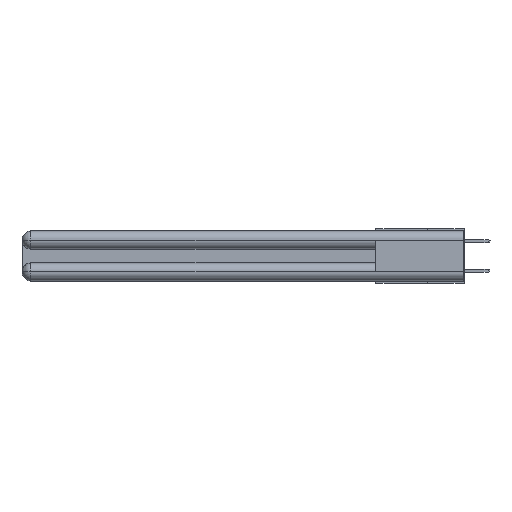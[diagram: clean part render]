
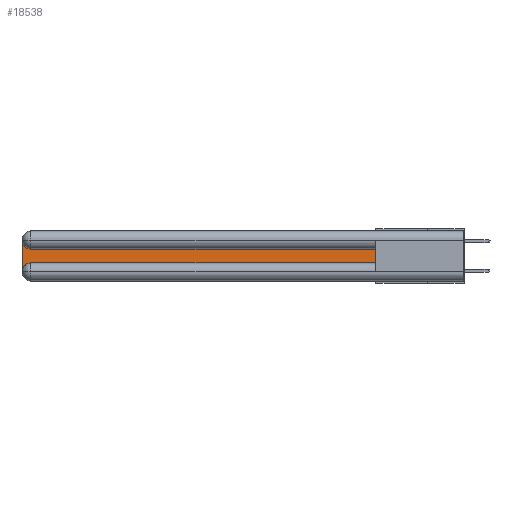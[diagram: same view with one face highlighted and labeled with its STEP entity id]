
A CAD part, left-side view. The second image highlights one B-rep face of the part: STEP entity #18538.
In plain terms, the highlighted planar face has unit normal (-1, 0, 0).
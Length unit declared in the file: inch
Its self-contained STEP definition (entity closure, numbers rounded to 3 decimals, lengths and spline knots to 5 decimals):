
#645 = EDGE_CURVE ( 'NONE', #24647, #4010, #3959, .T. ) ;
#1562 = VERTEX_POINT ( 'NONE', #2210 ) ;
#2210 = CARTESIAN_POINT ( 'NONE',  ( 0.075, 2.94, -0.1225 ) ) ;
#3118 = DIRECTION ( 'NONE',  ( 0., 1., 0. ) ) ;
#3959 = CIRCLE ( 'NONE', #5867, 0.06 ) ;
#4010 = VERTEX_POINT ( 'NONE', #17781 ) ;
#4594 = EDGE_CURVE ( 'NONE', #27675, #24647, #27883, .T. ) ;
#4763 = EDGE_CURVE ( 'NONE', #5570, #25290, #13779, .T. ) ;
#5570 = VERTEX_POINT ( 'NONE', #21222 ) ;
#5867 = AXIS2_PLACEMENT_3D ( 'NONE', #15861, #25127, #15965 ) ;
#6139 = CARTESIAN_POINT ( 'NONE',  ( 0.075, 0.6, -0.2175 ) ) ;
#8546 = VECTOR ( 'NONE', #24603, 39.37008 ) ;
#8799 = CARTESIAN_POINT ( 'NONE',  ( 0.075, 0.6, -0.2175 ) ) ;
#8911 = DIRECTION ( 'NONE',  ( 0., 0., -1. ) ) ;
#9016 = CARTESIAN_POINT ( 'NONE',  ( 0.075, 2.94, -0.0625 ) ) ;
#9846 = AXIS2_PLACEMENT_3D ( 'NONE', #9016, #16384, #8911 ) ;
#9885 = EDGE_CURVE ( 'NONE', #4010, #5570, #25580, .T. ) ;
#10174 = CIRCLE ( 'NONE', #9846, 0.06 ) ;
#11277 = VECTOR ( 'NONE', #3118, 39.37008 ) ;
#12378 = EDGE_LOOP ( 'NONE', ( #25102, #29614, #30507, #28700, #30766, #19799 ) ) ;
#13779 = LINE ( 'NONE', #6139, #19370 ) ;
#15055 = CARTESIAN_POINT ( 'NONE',  ( 0.075, 0.6, -0.1225 ) ) ;
#15650 = AXIS2_PLACEMENT_3D ( 'NONE', #21592, #26743, #17094 ) ;
#15861 = CARTESIAN_POINT ( 'NONE',  ( 0.075, 2.94, -0.2775 ) ) ;
#15965 = DIRECTION ( 'NONE',  ( 0., 0., -1. ) ) ;
#16384 = DIRECTION ( 'NONE',  ( 1., 0., 0. ) ) ;
#17094 = DIRECTION ( 'NONE',  ( 0., 0., -1. ) ) ;
#17781 = CARTESIAN_POINT ( 'NONE',  ( 0.075, 2.94, -0.2175 ) ) ;
#18175 = VECTOR ( 'NONE', #30383, 39.37008 ) ;
#18538 = ADVANCED_FACE ( 'NONE', ( #22203 ), #19207, .F. ) ;
#18780 = CARTESIAN_POINT ( 'NONE',  ( 0.075, 3., -0.2775 ) ) ;
#19207 = PLANE ( 'NONE',  #15650 ) ;
#19370 = VECTOR ( 'NONE', #27608, 39.37008 ) ;
#19799 = ORIENTED_EDGE ( 'NONE', *, *, #4763, .T. ) ;
#20204 = EDGE_CURVE ( 'NONE', #25290, #1562, #21694, .T. ) ;
#21222 = CARTESIAN_POINT ( 'NONE',  ( 0.075, 0.6, -0.2175 ) ) ;
#21592 = CARTESIAN_POINT ( 'NONE',  ( 0.075, 3., -0.1225 ) ) ;
#21694 = LINE ( 'NONE', #15055, #11277 ) ;
#21967 = CARTESIAN_POINT ( 'NONE',  ( 0.075, 0.6, -0.1225 ) ) ;
#22203 = FACE_OUTER_BOUND ( 'NONE', #12378, .T. ) ;
#24504 = CARTESIAN_POINT ( 'NONE',  ( 0.075, 3., -0.2175 ) ) ;
#24603 = DIRECTION ( 'NONE',  ( 0., 0., -1. ) ) ;
#24647 = VERTEX_POINT ( 'NONE', #18780 ) ;
#25102 = ORIENTED_EDGE ( 'NONE', *, *, #20204, .T. ) ;
#25127 = DIRECTION ( 'NONE',  ( 1., 0., 0. ) ) ;
#25290 = VERTEX_POINT ( 'NONE', #21967 ) ;
#25580 = LINE ( 'NONE', #8799, #18175 ) ;
#26321 = CARTESIAN_POINT ( 'NONE',  ( 0.075, 3., -0.0625 ) ) ;
#26743 = DIRECTION ( 'NONE',  ( 1., 0., 0. ) ) ;
#27047 = EDGE_CURVE ( 'NONE', #1562, #27675, #10174, .T. ) ;
#27608 = DIRECTION ( 'NONE',  ( 0., 0., 1. ) ) ;
#27675 = VERTEX_POINT ( 'NONE', #26321 ) ;
#27883 = LINE ( 'NONE', #24504, #8546 ) ;
#28700 = ORIENTED_EDGE ( 'NONE', *, *, #645, .T. ) ;
#29614 = ORIENTED_EDGE ( 'NONE', *, *, #27047, .T. ) ;
#30383 = DIRECTION ( 'NONE',  ( 0., -1., 0. ) ) ;
#30507 = ORIENTED_EDGE ( 'NONE', *, *, #4594, .T. ) ;
#30766 = ORIENTED_EDGE ( 'NONE', *, *, #9885, .T. ) ;
